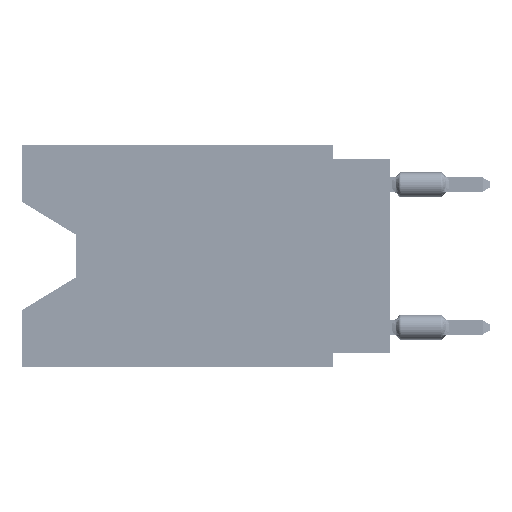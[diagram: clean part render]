
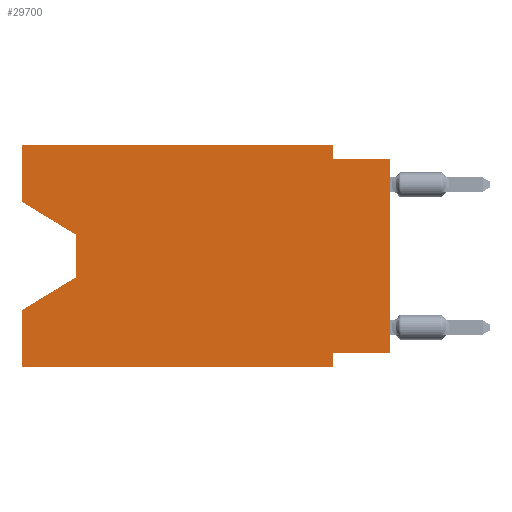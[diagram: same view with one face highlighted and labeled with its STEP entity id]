
A CAD part, left-side view. The second image highlights one B-rep face of the part: STEP entity #29700.
In plain terms, the highlighted planar face has unit normal (-1, 0, 0).
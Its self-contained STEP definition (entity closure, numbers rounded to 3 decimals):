
#973 = DIRECTION ( 'NONE',  ( 0., 0., 1. ) ) ;
#1074 = DIRECTION ( 'NONE',  ( 0., 0., -1. ) ) ;
#1764 = EDGE_CURVE ( 'NONE', #38072, #46757, #45367, .T. ) ;
#2052 = CARTESIAN_POINT ( 'NONE',  ( 0., 16.383, 0. ) ) ;
#2470 = VERTEX_POINT ( 'NONE', #64419 ) ;
#3016 = DIRECTION ( 'NONE',  ( 0., 0., 1. ) ) ;
#4167 = CARTESIAN_POINT ( 'NONE',  ( 0., 16.383, -7.36 ) ) ;
#4653 = VECTOR ( 'NONE', #3016, 1000. ) ;
#4701 = CARTESIAN_POINT ( 'NONE',  ( 0., 16.383, 0. ) ) ;
#5107 = DIRECTION ( 'NONE',  ( 0., -1., 0. ) ) ;
#7219 = LINE ( 'NONE', #66254, #58077 ) ;
#7463 = CARTESIAN_POINT ( 'NONE',  ( 0., 0., -9.271 ) ) ;
#8223 = VECTOR ( 'NONE', #9354, 1000. ) ;
#8279 = CARTESIAN_POINT ( 'NONE',  ( 0., 0., 0. ) ) ;
#8338 = CARTESIAN_POINT ( 'NONE',  ( 0., 13.97, -4.013 ) ) ;
#8679 = VECTOR ( 'NONE', #48170, 1000. ) ;
#8751 = VERTEX_POINT ( 'NONE', #45183 ) ;
#9071 = EDGE_CURVE ( 'NONE', #32234, #45127, #53834, .T. ) ;
#9354 = DIRECTION ( 'NONE',  ( 0., -1., 0. ) ) ;
#9512 = CARTESIAN_POINT ( 'NONE',  ( 0., 0., -9.271 ) ) ;
#10024 = CARTESIAN_POINT ( 'NONE',  ( 0., 16.383, 0. ) ) ;
#10259 = DIRECTION ( 'NONE',  ( 0., 0., 1. ) ) ;
#12452 = VERTEX_POINT ( 'NONE', #26796 ) ;
#12785 = VERTEX_POINT ( 'NONE', #16813 ) ;
#14898 = CARTESIAN_POINT ( 'NONE',  ( 0., 13.97, -5.893 ) ) ;
#15632 = ORIENTED_EDGE ( 'NONE', *, *, #19166, .F. ) ;
#16187 = EDGE_CURVE ( 'NONE', #36448, #12785, #56136, .T. ) ;
#16258 = VECTOR ( 'NONE', #51684, 1000. ) ;
#16813 = CARTESIAN_POINT ( 'NONE',  ( 0., 0., -0.635 ) ) ;
#16930 = CARTESIAN_POINT ( 'NONE',  ( 0., 13.97, -4.013 ) ) ;
#17075 = VECTOR ( 'NONE', #5107, 1000. ) ;
#17197 = DIRECTION ( 'NONE',  ( 0., 0.855, -0.519 ) ) ;
#17639 = VECTOR ( 'NONE', #973, 1000. ) ;
#19148 = VERTEX_POINT ( 'NONE', #4167 ) ;
#19166 = EDGE_CURVE ( 'NONE', #2470, #61681, #32087, .T. ) ;
#20077 = LINE ( 'NONE', #4701, #65641 ) ;
#20229 = ORIENTED_EDGE ( 'NONE', *, *, #55466, .F. ) ;
#20509 = CARTESIAN_POINT ( 'NONE',  ( 0., 16.383, -9.906 ) ) ;
#22154 = EDGE_LOOP ( 'NONE', ( #34145, #29328, #38217, #56009, #29783, #56608, #34126, #59168, #36005, #15632, #20229, #51322 ) ) ;
#25241 = DIRECTION ( 'NONE',  ( 0., 1., 0. ) ) ;
#26796 = CARTESIAN_POINT ( 'NONE',  ( 0., 16.383, -9.906 ) ) ;
#28068 = EDGE_CURVE ( 'NONE', #12452, #19148, #33464, .T. ) ;
#28382 = CARTESIAN_POINT ( 'NONE',  ( 0., 13.97, -5.893 ) ) ;
#28531 = DIRECTION ( 'NONE',  ( 0., -1., 0. ) ) ;
#28608 = DIRECTION ( 'NONE',  ( 1., 0., 0. ) ) ;
#29328 = ORIENTED_EDGE ( 'NONE', *, *, #1764, .T. ) ;
#29512 = CARTESIAN_POINT ( 'NONE',  ( 0., 2.54, -9.906 ) ) ;
#29700 = ADVANCED_FACE ( 'NONE', ( #40135 ), #61443, .F. ) ;
#29783 = ORIENTED_EDGE ( 'NONE', *, *, #57897, .T. ) ;
#30780 = CARTESIAN_POINT ( 'NONE',  ( 0., 16.383, -2.546 ) ) ;
#32087 = LINE ( 'NONE', #47145, #8679 ) ;
#32178 = CARTESIAN_POINT ( 'NONE',  ( 0., 2.54, -9.906 ) ) ;
#32234 = VERTEX_POINT ( 'NONE', #56529 ) ;
#32547 = EDGE_CURVE ( 'NONE', #61681, #12785, #7219, .T. ) ;
#33464 = LINE ( 'NONE', #54772, #17639 ) ;
#34126 = ORIENTED_EDGE ( 'NONE', *, *, #58710, .F. ) ;
#34145 = ORIENTED_EDGE ( 'NONE', *, *, #62619, .T. ) ;
#36005 = ORIENTED_EDGE ( 'NONE', *, *, #32547, .F. ) ;
#36448 = VERTEX_POINT ( 'NONE', #7463 ) ;
#38072 = VERTEX_POINT ( 'NONE', #16930 ) ;
#38134 = VERTEX_POINT ( 'NONE', #30780 ) ;
#38217 = ORIENTED_EDGE ( 'NONE', *, *, #49519, .T. ) ;
#40098 = AXIS2_PLACEMENT_3D ( 'NONE', #2052, #28608, #60033 ) ;
#40135 = FACE_OUTER_BOUND ( 'NONE', #22154, .T. ) ;
#40331 = CARTESIAN_POINT ( 'NONE',  ( 0., 2.54, -0.635 ) ) ;
#40482 = DIRECTION ( 'NONE',  ( 0., 0., -1. ) ) ;
#41850 = LINE ( 'NONE', #10024, #8223 ) ;
#43931 = VECTOR ( 'NONE', #25241, 1000. ) ;
#44806 = LINE ( 'NONE', #28382, #53221 ) ;
#45127 = VERTEX_POINT ( 'NONE', #29512 ) ;
#45183 = CARTESIAN_POINT ( 'NONE',  ( 0., 16.383, 0. ) ) ;
#45367 = LINE ( 'NONE', #8338, #54760 ) ;
#46225 = LINE ( 'NONE', #9512, #43931 ) ;
#46757 = VERTEX_POINT ( 'NONE', #14898 ) ;
#47145 = CARTESIAN_POINT ( 'NONE',  ( 0., 2.54, 0. ) ) ;
#47545 = VECTOR ( 'NONE', #1074, 1000. ) ;
#48170 = DIRECTION ( 'NONE',  ( 0., 0., -1. ) ) ;
#49519 = EDGE_CURVE ( 'NONE', #46757, #19148, #44806, .T. ) ;
#51322 = ORIENTED_EDGE ( 'NONE', *, *, #65811, .F. ) ;
#51684 = DIRECTION ( 'NONE',  ( 0., -0.855, -0.519 ) ) ;
#53221 = VECTOR ( 'NONE', #17197, 1000. ) ;
#53322 = LINE ( 'NONE', #20509, #17075 ) ;
#53834 = LINE ( 'NONE', #32178, #47545 ) ;
#54760 = VECTOR ( 'NONE', #40482, 1000. ) ;
#54772 = CARTESIAN_POINT ( 'NONE',  ( 0., 16.383, 0. ) ) ;
#55466 = EDGE_CURVE ( 'NONE', #8751, #2470, #41850, .T. ) ;
#56009 = ORIENTED_EDGE ( 'NONE', *, *, #28068, .F. ) ;
#56136 = LINE ( 'NONE', #8279, #4653 ) ;
#56529 = CARTESIAN_POINT ( 'NONE',  ( 0., 2.54, -9.271 ) ) ;
#56608 = ORIENTED_EDGE ( 'NONE', *, *, #9071, .F. ) ;
#57897 = EDGE_CURVE ( 'NONE', #12452, #45127, #53322, .T. ) ;
#58077 = VECTOR ( 'NONE', #28531, 1000. ) ;
#58710 = EDGE_CURVE ( 'NONE', #36448, #32234, #46225, .T. ) ;
#59168 = ORIENTED_EDGE ( 'NONE', *, *, #16187, .T. ) ;
#60033 = DIRECTION ( 'NONE',  ( 0., 0., -1. ) ) ;
#61103 = CARTESIAN_POINT ( 'NONE',  ( 0., 16.383, -2.546 ) ) ;
#61443 = PLANE ( 'NONE',  #40098 ) ;
#61681 = VERTEX_POINT ( 'NONE', #40331 ) ;
#62619 = EDGE_CURVE ( 'NONE', #38134, #38072, #66359, .T. ) ;
#64419 = CARTESIAN_POINT ( 'NONE',  ( 0., 2.54, 0. ) ) ;
#65641 = VECTOR ( 'NONE', #10259, 1000. ) ;
#65811 = EDGE_CURVE ( 'NONE', #38134, #8751, #20077, .T. ) ;
#66254 = CARTESIAN_POINT ( 'NONE',  ( 0., 0., -0.635 ) ) ;
#66359 = LINE ( 'NONE', #61103, #16258 ) ;
